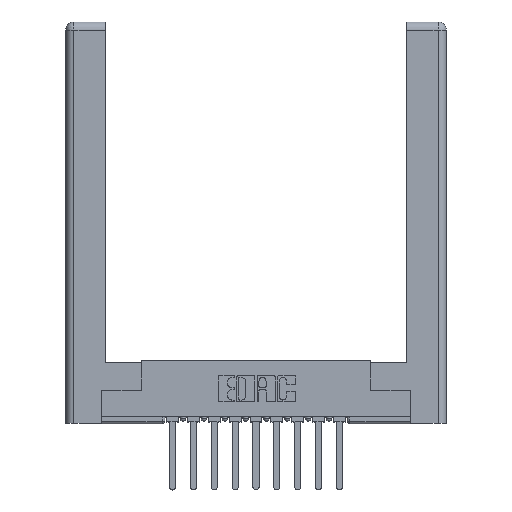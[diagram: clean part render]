
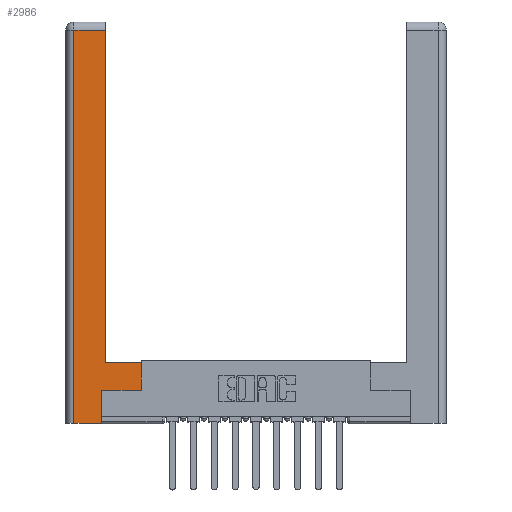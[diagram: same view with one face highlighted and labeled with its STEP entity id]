
A CAD part, top view. The second image highlights one B-rep face of the part: STEP entity #2986.
In plain terms, the highlighted planar face has unit normal (0, 0, 1).
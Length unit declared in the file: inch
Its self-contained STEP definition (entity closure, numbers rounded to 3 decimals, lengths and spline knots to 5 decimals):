
#33 = CARTESIAN_POINT ( 'NONE',  ( 0.265, 0.245, 0. ) ) ;
#377 = ORIENTED_EDGE ( 'NONE', *, *, #9411, .T. ) ;
#407 = CARTESIAN_POINT ( 'NONE',  ( 0.0615, 2.94, 0. ) ) ;
#514 = CARTESIAN_POINT ( 'NONE',  ( 0.565, 0.245, 0. ) ) ;
#607 = CARTESIAN_POINT ( 'NONE',  ( 0.295, 3., 0. ) ) ;
#998 = EDGE_CURVE ( 'NONE', #4252, #11361, #2997, .T. ) ;
#1226 = CARTESIAN_POINT ( 'NONE',  ( 0., 0., 0. ) ) ;
#1260 = VERTEX_POINT ( 'NONE', #11780 ) ;
#1332 = VECTOR ( 'NONE', #1695, 39.37008 ) ;
#1695 = DIRECTION ( 'NONE',  ( 1., 0., 0. ) ) ;
#1797 = ORIENTED_EDGE ( 'NONE', *, *, #2090, .T. ) ;
#1937 = ORIENTED_EDGE ( 'NONE', *, *, #4919, .T. ) ;
#1964 = DIRECTION ( 'NONE',  ( 0., 1., 0. ) ) ;
#2090 = EDGE_CURVE ( 'NONE', #11361, #8210, #4412, .T. ) ;
#2164 = LINE ( 'NONE', #4080, #5991 ) ;
#2423 = PLANE ( 'NONE',  #8730 ) ;
#2750 = LINE ( 'NONE', #407, #9718 ) ;
#2806 = CARTESIAN_POINT ( 'NONE',  ( 0.295, 0.45, 0. ) ) ;
#2986 = ADVANCED_FACE ( 'NONE', ( #5106 ), #2423, .F. ) ;
#2997 = LINE ( 'NONE', #514, #1332 ) ;
#3064 = VECTOR ( 'NONE', #4295, 39.37008 ) ;
#3196 = EDGE_CURVE ( 'NONE', #8766, #8732, #2750, .T. ) ;
#3650 = ORIENTED_EDGE ( 'NONE', *, *, #12595, .T. ) ;
#4080 = CARTESIAN_POINT ( 'NONE',  ( 0.295, 0.45, 0. ) ) ;
#4189 = DIRECTION ( 'NONE',  ( 0., -1., 0. ) ) ;
#4202 = CARTESIAN_POINT ( 'NONE',  ( 0.295, 2.94, 0. ) ) ;
#4252 = VERTEX_POINT ( 'NONE', #33 ) ;
#4295 = DIRECTION ( 'NONE',  ( 0., 1., 0. ) ) ;
#4412 = LINE ( 'NONE', #6805, #14672 ) ;
#4698 = LINE ( 'NONE', #6404, #14931 ) ;
#4919 = EDGE_CURVE ( 'NONE', #6076, #8766, #12372, .T. ) ;
#5106 = FACE_OUTER_BOUND ( 'NONE', #13188, .T. ) ;
#5991 = VECTOR ( 'NONE', #7455, 39.37008 ) ;
#6076 = VERTEX_POINT ( 'NONE', #2806 ) ;
#6185 = VECTOR ( 'NONE', #6568, 39.37008 ) ;
#6404 = CARTESIAN_POINT ( 'NONE',  ( 0.0615, 0., 0. ) ) ;
#6568 = DIRECTION ( 'NONE',  ( 1., 0., 0. ) ) ;
#6805 = CARTESIAN_POINT ( 'NONE',  ( 0.565, 0.45, 0. ) ) ;
#7001 = DIRECTION ( 'NONE',  ( -1., 0., 0. ) ) ;
#7097 = CARTESIAN_POINT ( 'NONE',  ( 0.265, 0., 0. ) ) ;
#7281 = EDGE_CURVE ( 'NONE', #8732, #1260, #4698, .T. ) ;
#7455 = DIRECTION ( 'NONE',  ( -1., 0., 0. ) ) ;
#7598 = ORIENTED_EDGE ( 'NONE', *, *, #7281, .T. ) ;
#7691 = CARTESIAN_POINT ( 'NONE',  ( 0.565, 0.45, 0. ) ) ;
#8210 = VERTEX_POINT ( 'NONE', #7691 ) ;
#8730 = AXIS2_PLACEMENT_3D ( 'NONE', #1226, #15085, #7001 ) ;
#8732 = VERTEX_POINT ( 'NONE', #9801 ) ;
#8766 = VERTEX_POINT ( 'NONE', #4202 ) ;
#9411 = EDGE_CURVE ( 'NONE', #12327, #4252, #9959, .T. ) ;
#9718 = VECTOR ( 'NONE', #9849, 39.37008 ) ;
#9801 = CARTESIAN_POINT ( 'NONE',  ( 0.0615, 2.94, 0. ) ) ;
#9849 = DIRECTION ( 'NONE',  ( -1., 0., 0. ) ) ;
#9913 = CARTESIAN_POINT ( 'NONE',  ( 0.565, 0.245, 0. ) ) ;
#9923 = DIRECTION ( 'NONE',  ( 0., 1., 0. ) ) ;
#9959 = LINE ( 'NONE', #12202, #13587 ) ;
#11361 = VERTEX_POINT ( 'NONE', #9913 ) ;
#11780 = CARTESIAN_POINT ( 'NONE',  ( 0.0615, 0., 0. ) ) ;
#12054 = ORIENTED_EDGE ( 'NONE', *, *, #3196, .T. ) ;
#12094 = EDGE_CURVE ( 'NONE', #1260, #12327, #12985, .T. ) ;
#12202 = CARTESIAN_POINT ( 'NONE',  ( 0.265, 0.245, 0. ) ) ;
#12327 = VERTEX_POINT ( 'NONE', #7097 ) ;
#12372 = LINE ( 'NONE', #607, #3064 ) ;
#12595 = EDGE_CURVE ( 'NONE', #8210, #6076, #2164, .T. ) ;
#12985 = LINE ( 'NONE', #14774, #6185 ) ;
#13188 = EDGE_LOOP ( 'NONE', ( #1937, #12054, #7598, #14115, #377, #15052, #1797, #3650 ) ) ;
#13587 = VECTOR ( 'NONE', #9923, 39.37008 ) ;
#14115 = ORIENTED_EDGE ( 'NONE', *, *, #12094, .T. ) ;
#14672 = VECTOR ( 'NONE', #1964, 39.37008 ) ;
#14774 = CARTESIAN_POINT ( 'NONE',  ( 0.265, 0., 0. ) ) ;
#14931 = VECTOR ( 'NONE', #4189, 39.37008 ) ;
#15052 = ORIENTED_EDGE ( 'NONE', *, *, #998, .T. ) ;
#15085 = DIRECTION ( 'NONE',  ( 0., 0., -1. ) ) ;
